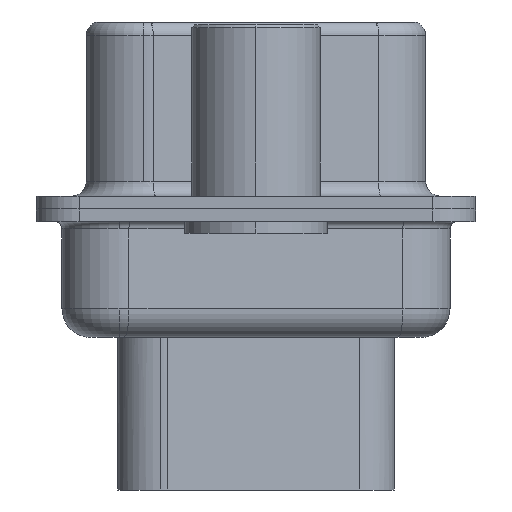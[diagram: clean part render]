
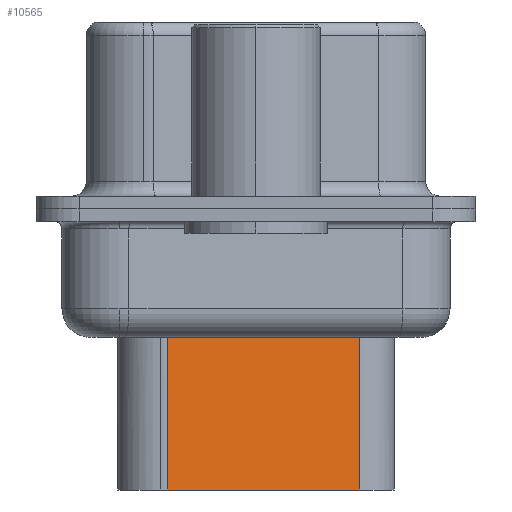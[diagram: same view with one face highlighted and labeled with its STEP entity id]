
A CAD part, left-side view. The second image highlights one B-rep face of the part: STEP entity #10565.
In plain terms, the highlighted planar face has unit normal (-0.985, -0.174, 0).
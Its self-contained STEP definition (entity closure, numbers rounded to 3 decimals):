
#570 = DIRECTION ( 'NONE',  ( -0.174, 0.985, 0. ) ) ;
#675 = CARTESIAN_POINT ( 'NONE',  ( 4.624, 3.09, -3.1 ) ) ;
#879 = LINE ( 'NONE', #15679, #19636 ) ;
#1857 = VECTOR ( 'NONE', #8061, 1000. ) ;
#2171 = VECTOR ( 'NONE', #570, 1000. ) ;
#2693 = CARTESIAN_POINT ( 'NONE',  ( 5.805, -3.61, -3.975 ) ) ;
#4832 = ORIENTED_EDGE ( 'NONE', *, *, #11993, .T. ) ;
#5711 = VERTEX_POINT ( 'NONE', #14828 ) ;
#6676 = PLANE ( 'NONE',  #13246 ) ;
#7436 = VERTEX_POINT ( 'NONE', #2693 ) ;
#7452 = LINE ( 'NONE', #32278, #13279 ) ;
#7706 = CARTESIAN_POINT ( 'NONE',  ( 4.624, 3.09, -3.975 ) ) ;
#8061 = DIRECTION ( 'NONE',  ( 0., 0., -1. ) ) ;
#8657 = DIRECTION ( 'NONE',  ( -0.985, -0.174, 0. ) ) ;
#10565 = ADVANCED_FACE ( 'NONE', ( #23948 ), #6676, .T. ) ;
#11993 = EDGE_CURVE ( 'NONE', #7436, #15039, #28337, .T. ) ;
#12220 = DIRECTION ( 'NONE',  ( -0.174, 0.985, 0. ) ) ;
#13063 = CARTESIAN_POINT ( 'NONE',  ( 4.453, 4.059, -3.975 ) ) ;
#13246 = AXIS2_PLACEMENT_3D ( 'NONE', #13919, #8657, #18861 ) ;
#13279 = VECTOR ( 'NONE', #12220, 1000. ) ;
#13919 = CARTESIAN_POINT ( 'NONE',  ( 4.624, 3.09, -3.1 ) ) ;
#14275 = CARTESIAN_POINT ( 'NONE',  ( 5.805, -3.61, -9.85 ) ) ;
#14828 = CARTESIAN_POINT ( 'NONE',  ( 4.624, 3.09, -9.85 ) ) ;
#15039 = VERTEX_POINT ( 'NONE', #7706 ) ;
#15679 = CARTESIAN_POINT ( 'NONE',  ( 5.805, -3.61, -3.1 ) ) ;
#16271 = EDGE_LOOP ( 'NONE', ( #28399, #4832, #17599, #18062 ) ) ;
#16448 = VERTEX_POINT ( 'NONE', #14275 ) ;
#17599 = ORIENTED_EDGE ( 'NONE', *, *, #32171, .T. ) ;
#18062 = ORIENTED_EDGE ( 'NONE', *, *, #21339, .F. ) ;
#18164 = DIRECTION ( 'NONE',  ( 0., 0., -1. ) ) ;
#18861 = DIRECTION ( 'NONE',  ( 0.174, -0.985, 0. ) ) ;
#19636 = VECTOR ( 'NONE', #18164, 1000. ) ;
#21339 = EDGE_CURVE ( 'NONE', #16448, #5711, #7452, .T. ) ;
#23352 = LINE ( 'NONE', #675, #1857 ) ;
#23948 = FACE_OUTER_BOUND ( 'NONE', #16271, .T. ) ;
#26453 = EDGE_CURVE ( 'NONE', #7436, #16448, #879, .T. ) ;
#28337 = LINE ( 'NONE', #13063, #2171 ) ;
#28399 = ORIENTED_EDGE ( 'NONE', *, *, #26453, .F. ) ;
#32171 = EDGE_CURVE ( 'NONE', #15039, #5711, #23352, .T. ) ;
#32278 = CARTESIAN_POINT ( 'NONE',  ( 4.624, 3.09, -9.85 ) ) ;
